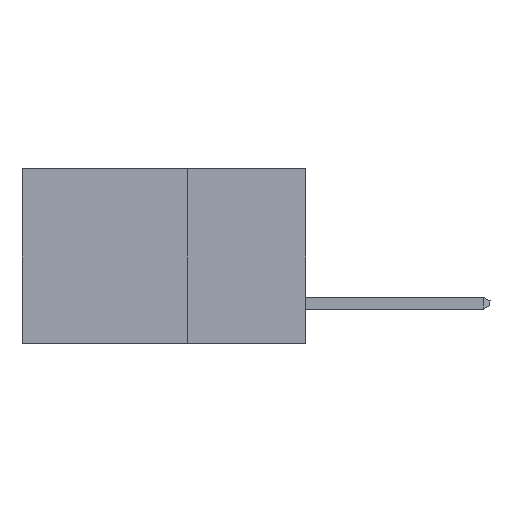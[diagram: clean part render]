
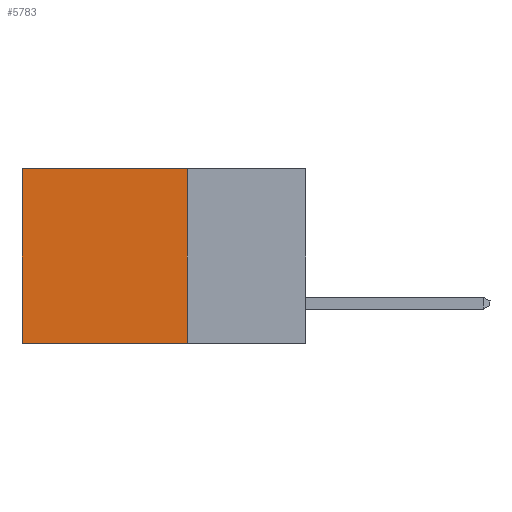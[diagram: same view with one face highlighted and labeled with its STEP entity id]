
A CAD part, left-side view. The second image highlights one B-rep face of the part: STEP entity #5783.
In plain terms, the highlighted planar face has unit normal (-1, 0, 0).
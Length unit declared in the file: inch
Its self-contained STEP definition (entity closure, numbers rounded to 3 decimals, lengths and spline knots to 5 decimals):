
#1333 = VERTEX_POINT ( 'NONE', #8494 ) ;
#1698 = FACE_OUTER_BOUND ( 'NONE', #13739, .T. ) ;
#2137 = CARTESIAN_POINT ( 'NONE',  ( 0.2615, 0.6, 0. ) ) ;
#2686 = CARTESIAN_POINT ( 'NONE',  ( 0.2615, 0.25, 0. ) ) ;
#2925 = CARTESIAN_POINT ( 'NONE',  ( 0.2615, 0.25, -0.37 ) ) ;
#3710 = CARTESIAN_POINT ( 'NONE',  ( 0.2615, 0.6, -0.37 ) ) ;
#4036 = EDGE_CURVE ( 'NONE', #1333, #18878, #4407, .T. ) ;
#4407 = LINE ( 'NONE', #11968, #13795 ) ;
#4723 = LINE ( 'NONE', #19711, #22234 ) ;
#4877 = VERTEX_POINT ( 'NONE', #22724 ) ;
#5783 = ADVANCED_FACE ( 'NONE', ( #1698 ), #13058, .F. ) ;
#6498 = EDGE_CURVE ( 'NONE', #20353, #18878, #4723, .T. ) ;
#7358 = DIRECTION ( 'NONE',  ( 0., 0., -1. ) ) ;
#8494 = CARTESIAN_POINT ( 'NONE',  ( 0.2615, 0.25, -0.37 ) ) ;
#8581 = ORIENTED_EDGE ( 'NONE', *, *, #18520, .F. ) ;
#9209 = DIRECTION ( 'NONE',  ( 1., 0., 0. ) ) ;
#9317 = VECTOR ( 'NONE', #18017, 39.37008 ) ;
#9836 = ORIENTED_EDGE ( 'NONE', *, *, #14150, .T. ) ;
#11968 = CARTESIAN_POINT ( 'NONE',  ( 0.2615, 0.25, -0.37 ) ) ;
#12339 = LINE ( 'NONE', #2925, #9317 ) ;
#12707 = ORIENTED_EDGE ( 'NONE', *, *, #4036, .F. ) ;
#13058 = PLANE ( 'NONE',  #18566 ) ;
#13739 = EDGE_LOOP ( 'NONE', ( #20958, #12707, #8581, #9836 ) ) ;
#13795 = VECTOR ( 'NONE', #19504, 39.37008 ) ;
#14150 = EDGE_CURVE ( 'NONE', #4877, #20353, #15519, .T. ) ;
#15499 = VECTOR ( 'NONE', #23140, 39.37008 ) ;
#15519 = LINE ( 'NONE', #2686, #15499 ) ;
#18017 = DIRECTION ( 'NONE',  ( 0., 0., -1. ) ) ;
#18505 = CARTESIAN_POINT ( 'NONE',  ( 0.2615, 0.25, -0.37 ) ) ;
#18520 = EDGE_CURVE ( 'NONE', #4877, #1333, #12339, .T. ) ;
#18566 = AXIS2_PLACEMENT_3D ( 'NONE', #18505, #9209, #7358 ) ;
#18878 = VERTEX_POINT ( 'NONE', #3710 ) ;
#19504 = DIRECTION ( 'NONE',  ( 0., 1., 0. ) ) ;
#19711 = CARTESIAN_POINT ( 'NONE',  ( 0.2615, 0.6, -0.37 ) ) ;
#20353 = VERTEX_POINT ( 'NONE', #2137 ) ;
#20958 = ORIENTED_EDGE ( 'NONE', *, *, #6498, .T. ) ;
#21950 = DIRECTION ( 'NONE',  ( 0., 0., -1. ) ) ;
#22234 = VECTOR ( 'NONE', #21950, 39.37008 ) ;
#22724 = CARTESIAN_POINT ( 'NONE',  ( 0.2615, 0.25, 0. ) ) ;
#23140 = DIRECTION ( 'NONE',  ( 0., 1., 0. ) ) ;
